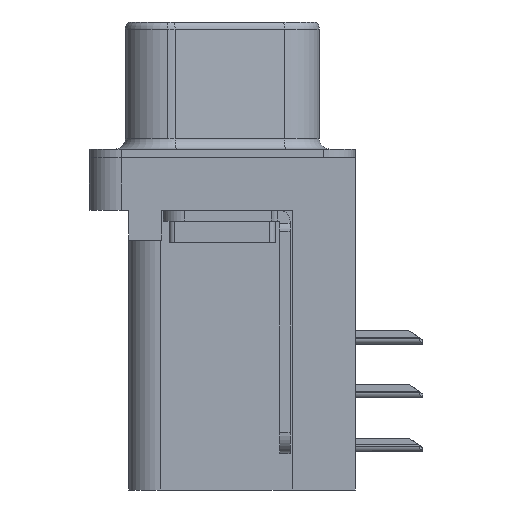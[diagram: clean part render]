
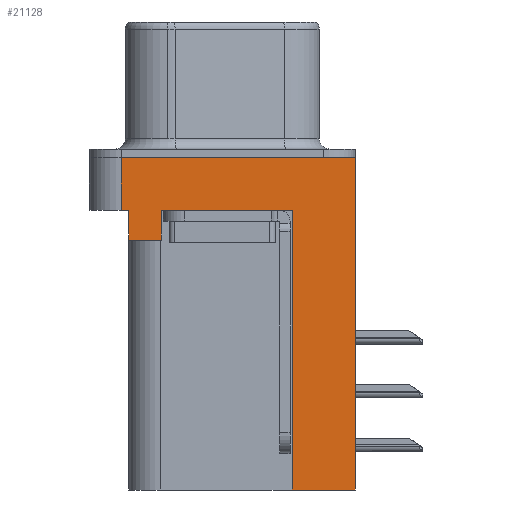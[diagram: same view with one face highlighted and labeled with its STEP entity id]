
A CAD part, left-side view. The second image highlights one B-rep face of the part: STEP entity #21128.
In plain terms, the highlighted planar face has unit normal (-1, 0, 0).
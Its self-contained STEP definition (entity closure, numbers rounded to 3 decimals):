
#451 = CARTESIAN_POINT ( 'NONE',  ( -2.91, -6.275, 0. ) ) ;
#584 = DIRECTION ( 'NONE',  ( -1., 0., 0. ) ) ;
#729 = ORIENTED_EDGE ( 'NONE', *, *, #8898, .F. ) ;
#2173 = VERTEX_POINT ( 'NONE', #34721 ) ;
#2350 = CARTESIAN_POINT ( 'NONE',  ( -2.91, -3.295, -2.5 ) ) ;
#2691 = CARTESIAN_POINT ( 'NONE',  ( -2.91, -6.275, -2.5 ) ) ;
#2932 = ORIENTED_EDGE ( 'NONE', *, *, #7933, .T. ) ;
#3693 = FACE_OUTER_BOUND ( 'NONE', #21250, .T. ) ;
#4372 = ORIENTED_EDGE ( 'NONE', *, *, #8835, .F. ) ;
#4784 = ORIENTED_EDGE ( 'NONE', *, *, #8849, .F. ) ;
#4955 = VERTEX_POINT ( 'NONE', #29188 ) ;
#4961 = ORIENTED_EDGE ( 'NONE', *, *, #8746, .F. ) ;
#6304 = ORIENTED_EDGE ( 'NONE', *, *, #8623, .T. ) ;
#6432 = ORIENTED_EDGE ( 'NONE', *, *, #8901, .F. ) ;
#6724 = DIRECTION ( 'NONE',  ( 0., 0., 1. ) ) ;
#6828 = VERTEX_POINT ( 'NONE', #21299 ) ;
#7933 = EDGE_CURVE ( 'NONE', #13030, #27679, #20713, .T. ) ;
#7955 = VECTOR ( 'NONE', #12247, 1000. ) ;
#7989 = CARTESIAN_POINT ( 'NONE',  ( -2.91, 4.425, -2.5 ) ) ;
#8077 = LINE ( 'NONE', #30383, #7955 ) ;
#8078 = CARTESIAN_POINT ( 'NONE',  ( -2.91, -6.275, -2.5 ) ) ;
#8174 = EDGE_CURVE ( 'NONE', #6828, #13030, #19513, .T. ) ;
#8467 = EDGE_CURVE ( 'NONE', #6828, #21640, #17311, .T. ) ;
#8623 = EDGE_CURVE ( 'NONE', #30700, #25059, #16572, .T. ) ;
#8671 = DIRECTION ( 'NONE',  ( 0., -1., 0. ) ) ;
#8746 = EDGE_CURVE ( 'NONE', #2173, #34439, #15696, .T. ) ;
#8835 = EDGE_CURVE ( 'NONE', #30700, #2173, #15281, .T. ) ;
#8849 = EDGE_CURVE ( 'NONE', #21640, #25059, #15213, .T. ) ;
#8898 = EDGE_CURVE ( 'NONE', #4955, #27679, #14949, .T. ) ;
#8901 = EDGE_CURVE ( 'NONE', #34916, #4955, #14863, .T. ) ;
#9313 = CARTESIAN_POINT ( 'NONE',  ( -2.91, 4.425, -3.9 ) ) ;
#9449 = CARTESIAN_POINT ( 'NONE',  ( -2.91, -6.275, -2.5 ) ) ;
#10260 = EDGE_CURVE ( 'NONE', #34916, #34439, #8077, .T. ) ;
#12247 = DIRECTION ( 'NONE',  ( 0., 0., 1. ) ) ;
#13030 = VERTEX_POINT ( 'NONE', #24914 ) ;
#14487 = DIRECTION ( 'NONE',  ( 0., 0., 1. ) ) ;
#14777 = VECTOR ( 'NONE', #22880, 1000. ) ;
#14843 = VECTOR ( 'NONE', #33159, 1000. ) ;
#14863 = LINE ( 'NONE', #20210, #14777 ) ;
#14949 = LINE ( 'NONE', #28019, #14843 ) ;
#15067 = VECTOR ( 'NONE', #32942, 1000. ) ;
#15213 = LINE ( 'NONE', #17462, #15067 ) ;
#15271 = VECTOR ( 'NONE', #6724, 1000. ) ;
#15281 = LINE ( 'NONE', #27812, #15271 ) ;
#15664 = VECTOR ( 'NONE', #32622, 1000. ) ;
#15696 = LINE ( 'NONE', #30063, #15664 ) ;
#16431 = VECTOR ( 'NONE', #8671, 1000. ) ;
#16572 = LINE ( 'NONE', #2691, #16431 ) ;
#17251 = VECTOR ( 'NONE', #33972, 1000. ) ;
#17311 = LINE ( 'NONE', #31414, #17251 ) ;
#17462 = CARTESIAN_POINT ( 'NONE',  ( -2.91, 4.425, -3.9 ) ) ;
#18198 = AXIS2_PLACEMENT_3D ( 'NONE', #9449, #584, #19965 ) ;
#19174 = VECTOR ( 'NONE', #14487, 1000. ) ;
#19513 = LINE ( 'NONE', #32431, #19174 ) ;
#19965 = DIRECTION ( 'NONE',  ( 0., 0., 1. ) ) ;
#20210 = CARTESIAN_POINT ( 'NONE',  ( -2.91, -3.295, -15.7 ) ) ;
#20516 = VECTOR ( 'NONE', #28995, 1000. ) ;
#20713 = LINE ( 'NONE', #8078, #20516 ) ;
#20812 = ORIENTED_EDGE ( 'NONE', *, *, #8174, .T. ) ;
#20942 = ORIENTED_EDGE ( 'NONE', *, *, #8467, .F. ) ;
#21128 = ADVANCED_FACE ( 'NONE', ( #3693 ), #30378, .T. ) ;
#21229 = CARTESIAN_POINT ( 'NONE',  ( -2.91, 4.775, -2.5 ) ) ;
#21250 = EDGE_LOOP ( 'NONE', ( #4961, #4372, #6304, #4784, #20942, #20812, #2932, #729, #6432, #24219 ) ) ;
#21299 = CARTESIAN_POINT ( 'NONE',  ( -2.91, 2.895, -3.9 ) ) ;
#21640 = VERTEX_POINT ( 'NONE', #9313 ) ;
#22880 = DIRECTION ( 'NONE',  ( 0., 1., 0. ) ) ;
#24219 = ORIENTED_EDGE ( 'NONE', *, *, #10260, .T. ) ;
#24914 = CARTESIAN_POINT ( 'NONE',  ( -2.91, 2.895, -2.5 ) ) ;
#25059 = VERTEX_POINT ( 'NONE', #7989 ) ;
#27679 = VERTEX_POINT ( 'NONE', #2350 ) ;
#27812 = CARTESIAN_POINT ( 'NONE',  ( -2.91, 4.775, -2.5 ) ) ;
#28019 = CARTESIAN_POINT ( 'NONE',  ( -2.91, -3.295, -15.7 ) ) ;
#28995 = DIRECTION ( 'NONE',  ( 0., -1., 0. ) ) ;
#29188 = CARTESIAN_POINT ( 'NONE',  ( -2.91, -3.295, -15.7 ) ) ;
#29385 = CARTESIAN_POINT ( 'NONE',  ( -2.91, -6.275, -15.7 ) ) ;
#30063 = CARTESIAN_POINT ( 'NONE',  ( -2.91, -6.275, 0. ) ) ;
#30378 = PLANE ( 'NONE',  #18198 ) ;
#30383 = CARTESIAN_POINT ( 'NONE',  ( -2.91, -6.275, -2.5 ) ) ;
#30700 = VERTEX_POINT ( 'NONE', #21229 ) ;
#31414 = CARTESIAN_POINT ( 'NONE',  ( -2.91, 4.425, -3.9 ) ) ;
#32431 = CARTESIAN_POINT ( 'NONE',  ( -2.91, 2.895, -3.9 ) ) ;
#32622 = DIRECTION ( 'NONE',  ( 0., -1., 0. ) ) ;
#32942 = DIRECTION ( 'NONE',  ( 0., 0., 1. ) ) ;
#33159 = DIRECTION ( 'NONE',  ( 0., 0., 1. ) ) ;
#33972 = DIRECTION ( 'NONE',  ( 0., 1., 0. ) ) ;
#34439 = VERTEX_POINT ( 'NONE', #451 ) ;
#34721 = CARTESIAN_POINT ( 'NONE',  ( -2.91, 4.775, 0. ) ) ;
#34916 = VERTEX_POINT ( 'NONE', #29385 ) ;
